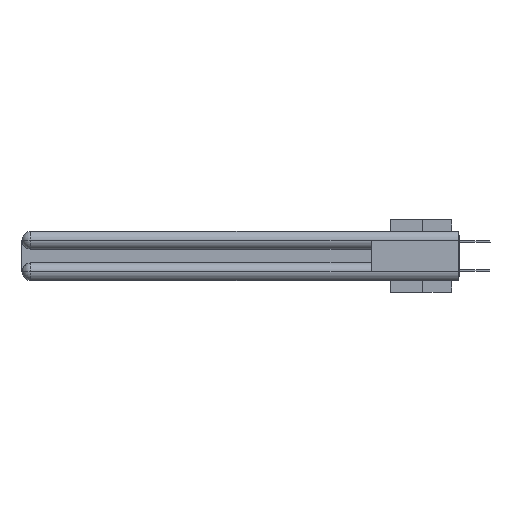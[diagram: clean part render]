
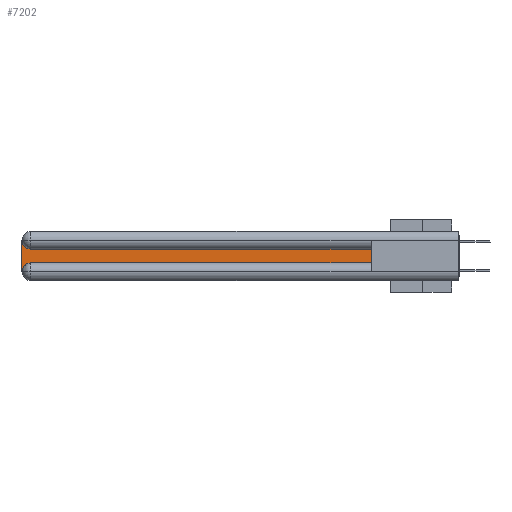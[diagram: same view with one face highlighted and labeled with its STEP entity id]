
A CAD part, left-side view. The second image highlights one B-rep face of the part: STEP entity #7202.
In plain terms, the highlighted planar face has unit normal (-1, 0, 0).
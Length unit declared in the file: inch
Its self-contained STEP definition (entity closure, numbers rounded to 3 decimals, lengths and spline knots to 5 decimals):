
#77 = DIRECTION ( 'NONE',  ( 1., 0., 0. ) ) ;
#884 = CARTESIAN_POINT ( 'NONE',  ( 0.075, 0.6, -0.2175 ) ) ;
#1070 = DIRECTION ( 'NONE',  ( 0., 0., -1. ) ) ;
#1329 = AXIS2_PLACEMENT_3D ( 'NONE', #24412, #30534, #24972 ) ;
#3255 = DIRECTION ( 'NONE',  ( 0., 0., -1. ) ) ;
#3525 = VERTEX_POINT ( 'NONE', #6203 ) ;
#3727 = FACE_OUTER_BOUND ( 'NONE', #9382, .T. ) ;
#5079 = ORIENTED_EDGE ( 'NONE', *, *, #15078, .T. ) ;
#5353 = AXIS2_PLACEMENT_3D ( 'NONE', #14935, #77, #8876 ) ;
#6040 = VECTOR ( 'NONE', #11506, 39.37008 ) ;
#6157 = CARTESIAN_POINT ( 'NONE',  ( 0.075, 3., -0.2175 ) ) ;
#6203 = CARTESIAN_POINT ( 'NONE',  ( 0.075, 3., -0.0625 ) ) ;
#6350 = VERTEX_POINT ( 'NONE', #32407 ) ;
#6794 = ORIENTED_EDGE ( 'NONE', *, *, #13238, .T. ) ;
#6900 = AXIS2_PLACEMENT_3D ( 'NONE', #12327, #27193, #1070 ) ;
#7202 = ADVANCED_FACE ( 'NONE', ( #3727 ), #30262, .F. ) ;
#7340 = CARTESIAN_POINT ( 'NONE',  ( 0.075, 2.94, -0.1225 ) ) ;
#7801 = ORIENTED_EDGE ( 'NONE', *, *, #12055, .T. ) ;
#8189 = CARTESIAN_POINT ( 'NONE',  ( 0.075, 0.6, -0.1225 ) ) ;
#8526 = EDGE_CURVE ( 'NONE', #23189, #23018, #35810, .T. ) ;
#8673 = CIRCLE ( 'NONE', #1329, 0.06 ) ;
#8876 = DIRECTION ( 'NONE',  ( 0., 0., -1. ) ) ;
#9047 = VERTEX_POINT ( 'NONE', #7340 ) ;
#9382 = EDGE_LOOP ( 'NONE', ( #9864, #7801, #5079, #6794, #11166, #16816 ) ) ;
#9864 = ORIENTED_EDGE ( 'NONE', *, *, #19596, .T. ) ;
#10152 = LINE ( 'NONE', #12810, #36342 ) ;
#11156 = VECTOR ( 'NONE', #3255, 39.37008 ) ;
#11166 = ORIENTED_EDGE ( 'NONE', *, *, #33260, .T. ) ;
#11506 = DIRECTION ( 'NONE',  ( 0., -1., 0. ) ) ;
#12055 = EDGE_CURVE ( 'NONE', #9047, #3525, #8673, .T. ) ;
#12269 = LINE ( 'NONE', #20273, #6040 ) ;
#12327 = CARTESIAN_POINT ( 'NONE',  ( 0.075, 3., -0.1225 ) ) ;
#12810 = CARTESIAN_POINT ( 'NONE',  ( 0.075, 0.6, -0.1225 ) ) ;
#13238 = EDGE_CURVE ( 'NONE', #18642, #6350, #21828, .T. ) ;
#13831 = CARTESIAN_POINT ( 'NONE',  ( 0.075, 3., -0.2775 ) ) ;
#14935 = CARTESIAN_POINT ( 'NONE',  ( 0.075, 2.94, -0.2775 ) ) ;
#15078 = EDGE_CURVE ( 'NONE', #3525, #18642, #32299, .T. ) ;
#16816 = ORIENTED_EDGE ( 'NONE', *, *, #8526, .T. ) ;
#18231 = DIRECTION ( 'NONE',  ( 0., 0., 1. ) ) ;
#18642 = VERTEX_POINT ( 'NONE', #13831 ) ;
#19596 = EDGE_CURVE ( 'NONE', #23018, #9047, #10152, .T. ) ;
#20273 = CARTESIAN_POINT ( 'NONE',  ( 0.075, 0.6, -0.2175 ) ) ;
#21828 = CIRCLE ( 'NONE', #5353, 0.06 ) ;
#23018 = VERTEX_POINT ( 'NONE', #8189 ) ;
#23189 = VERTEX_POINT ( 'NONE', #26671 ) ;
#24412 = CARTESIAN_POINT ( 'NONE',  ( 0.075, 2.94, -0.0625 ) ) ;
#24972 = DIRECTION ( 'NONE',  ( 0., 0., -1. ) ) ;
#26671 = CARTESIAN_POINT ( 'NONE',  ( 0.075, 0.6, -0.2175 ) ) ;
#27193 = DIRECTION ( 'NONE',  ( 1., 0., 0. ) ) ;
#30181 = DIRECTION ( 'NONE',  ( 0., 1., 0. ) ) ;
#30262 = PLANE ( 'NONE',  #6900 ) ;
#30534 = DIRECTION ( 'NONE',  ( 1., 0., 0. ) ) ;
#30931 = VECTOR ( 'NONE', #18231, 39.37008 ) ;
#32299 = LINE ( 'NONE', #6157, #11156 ) ;
#32407 = CARTESIAN_POINT ( 'NONE',  ( 0.075, 2.94, -0.2175 ) ) ;
#33260 = EDGE_CURVE ( 'NONE', #6350, #23189, #12269, .T. ) ;
#35810 = LINE ( 'NONE', #884, #30931 ) ;
#36342 = VECTOR ( 'NONE', #30181, 39.37008 ) ;
